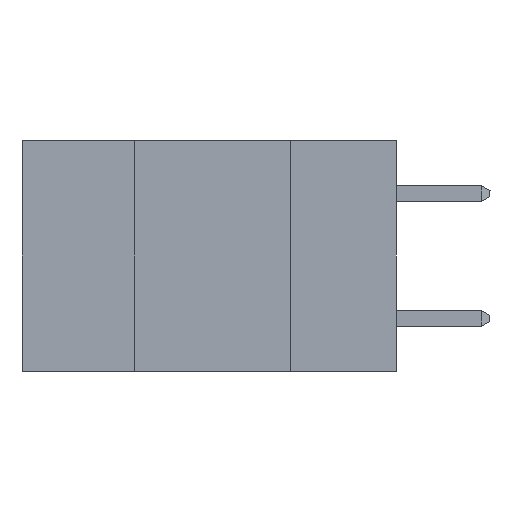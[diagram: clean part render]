
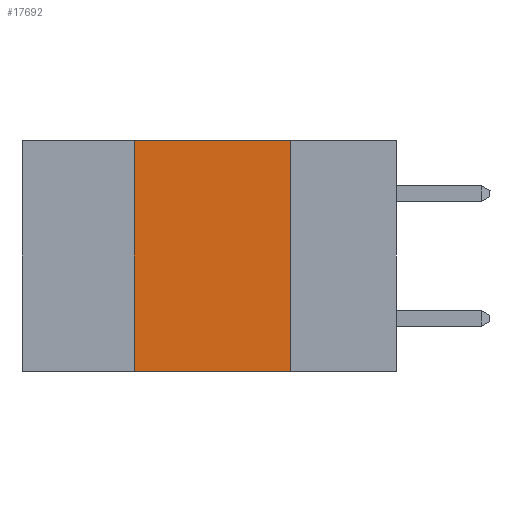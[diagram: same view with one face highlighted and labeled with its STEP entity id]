
A CAD part, left-side view. The second image highlights one B-rep face of the part: STEP entity #17692.
In plain terms, the highlighted planar face has unit normal (-1, 0, 0).
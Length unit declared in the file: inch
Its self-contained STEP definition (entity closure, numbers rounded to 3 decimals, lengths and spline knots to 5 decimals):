
#1248 = DIRECTION ( 'NONE',  ( 1., 0., 0. ) ) ;
#1310 = EDGE_LOOP ( 'NONE', ( #23504, #17416, #18198, #14127 ) ) ;
#1317 = VERTEX_POINT ( 'NONE', #20167 ) ;
#1658 = VECTOR ( 'NONE', #3643, 39.37008 ) ;
#1766 = VECTOR ( 'NONE', #11449, 39.37008 ) ;
#2347 = FACE_OUTER_BOUND ( 'NONE', #1310, .T. ) ;
#2764 = LINE ( 'NONE', #16893, #12107 ) ;
#3399 = VERTEX_POINT ( 'NONE', #21795 ) ;
#3643 = DIRECTION ( 'NONE',  ( 0., 0., 1. ) ) ;
#3664 = EDGE_CURVE ( 'NONE', #5880, #17100, #2764, .T. ) ;
#4041 = CARTESIAN_POINT ( 'NONE',  ( 0., 0.6, -0.37 ) ) ;
#4118 = LINE ( 'NONE', #6132, #22811 ) ;
#5880 = VERTEX_POINT ( 'NONE', #8735 ) ;
#6132 = CARTESIAN_POINT ( 'NONE',  ( 0., 0.17, -0.37 ) ) ;
#6206 = LINE ( 'NONE', #4041, #1766 ) ;
#6667 = LINE ( 'NONE', #14794, #1658 ) ;
#6849 = PLANE ( 'NONE',  #12270 ) ;
#8735 = CARTESIAN_POINT ( 'NONE',  ( 0., 0.42, 0. ) ) ;
#8996 = CARTESIAN_POINT ( 'NONE',  ( 0., 0.17, 0. ) ) ;
#11236 = DIRECTION ( 'NONE',  ( 0., -1., 0. ) ) ;
#11449 = DIRECTION ( 'NONE',  ( 0., -1., 0. ) ) ;
#12107 = VECTOR ( 'NONE', #11236, 39.37008 ) ;
#12270 = AXIS2_PLACEMENT_3D ( 'NONE', #12446, #1248, #14335 ) ;
#12446 = CARTESIAN_POINT ( 'NONE',  ( 0., 0.6, 0. ) ) ;
#14127 = ORIENTED_EDGE ( 'NONE', *, *, #16655, .T. ) ;
#14335 = DIRECTION ( 'NONE',  ( 0., 0., -1. ) ) ;
#14794 = CARTESIAN_POINT ( 'NONE',  ( 0., 0.42, -0.37 ) ) ;
#16655 = EDGE_CURVE ( 'NONE', #3399, #1317, #6206, .T. ) ;
#16893 = CARTESIAN_POINT ( 'NONE',  ( 0., 0.6, 0. ) ) ;
#17100 = VERTEX_POINT ( 'NONE', #8996 ) ;
#17416 = ORIENTED_EDGE ( 'NONE', *, *, #3664, .F. ) ;
#17426 = EDGE_CURVE ( 'NONE', #17100, #1317, #4118, .T. ) ;
#17692 = ADVANCED_FACE ( 'NONE', ( #2347 ), #6849, .F. ) ;
#18198 = ORIENTED_EDGE ( 'NONE', *, *, #24150, .F. ) ;
#20167 = CARTESIAN_POINT ( 'NONE',  ( 0., 0.17, -0.37 ) ) ;
#21082 = DIRECTION ( 'NONE',  ( 0., 0., -1. ) ) ;
#21795 = CARTESIAN_POINT ( 'NONE',  ( 0., 0.42, -0.37 ) ) ;
#22811 = VECTOR ( 'NONE', #21082, 39.37008 ) ;
#23504 = ORIENTED_EDGE ( 'NONE', *, *, #17426, .F. ) ;
#24150 = EDGE_CURVE ( 'NONE', #3399, #5880, #6667, .T. ) ;
